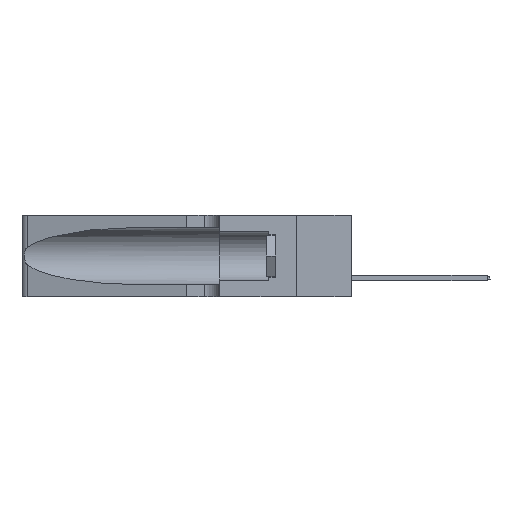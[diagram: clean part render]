
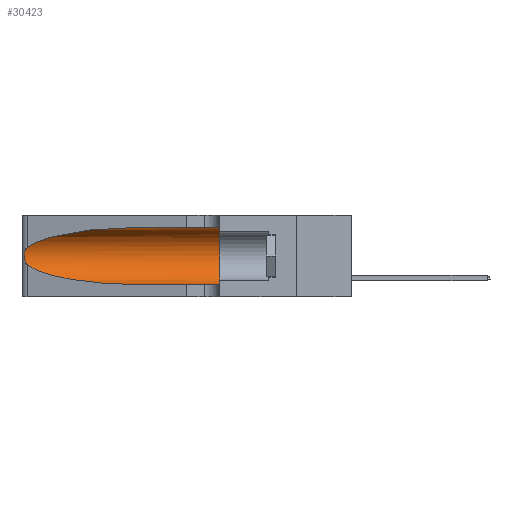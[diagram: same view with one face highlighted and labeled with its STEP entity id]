
A CAD part, left-side view. The second image highlights one B-rep face of the part: STEP entity #30423.
In plain terms, the highlighted cylindrical face has radius 3.308 mm (diameter 6.617 mm), a partial arc.
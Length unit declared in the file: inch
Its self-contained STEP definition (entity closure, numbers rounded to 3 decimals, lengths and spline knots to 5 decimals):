
#469 = VERTEX_POINT ( 'NONE', #9005 ) ;
#477 = CARTESIAN_POINT ( 'NONE',  ( 0.1305, 1.61858, 0.185 ) ) ;
#2237 = CARTESIAN_POINT ( 'NONE',  ( 0.1305, 0.72297, 0.31525 ) ) ;
#2876 = AXIS2_PLACEMENT_3D ( 'NONE', #477, #12611, #15053 ) ;
#3534 = CARTESIAN_POINT ( 'NONE',  ( 0.1305, 0.72297, 0.05475 ) ) ;
#3606 = CIRCLE ( 'NONE', #16011, 0.13025 ) ;
#4184 = CARTESIAN_POINT ( 'NONE',  ( 0.25555, 1.22993, 0.14849 ) ) ;
#4332 = CARTESIAN_POINT ( 'NONE',  ( 0.18966, 0.96281, 0.31525 ) ) ;
#4668 = CYLINDRICAL_SURFACE ( 'NONE', #2876, 0.13025 ) ;
#5025 = DIRECTION ( 'NONE',  ( 0., -1., 0. ) ) ;
#5222 = ORIENTED_EDGE ( 'NONE', *, *, #16551, .T. ) ;
#5290 = EDGE_CURVE ( 'NONE', #26591, #16849, #30680, .T. ) ;
#5317 = CARTESIAN_POINT ( 'NONE',  ( 0.25787, 1.23484, 0.2124 ) ) ;
#5686 = VECTOR ( 'NONE', #14224, 39.37008 ) ;
#5918 = B_SPLINE_CURVE_WITH_KNOTS ( 'NONE', 3,
 ( #22408, #17344, #20096, #5317, #20200, #22194, #24714, #27109, #20003, #15040, #16251, #17887, #4184, #11482 ),
 .UNSPECIFIED., .F., .F.,
 ( 4, 2, 2, 2, 2, 2, 4 ),
 ( 0., 0.00027, 0.00053, 0.00107, 0.0016, 0.00187, 0.00214 ),
 .UNSPECIFIED. ) ;
#6559 = EDGE_LOOP ( 'NONE', ( #10654, #5222, #26106, #30588, #6866, #19528 ) ) ;
#6730 = CARTESIAN_POINT ( 'NONE',  ( 0.1305, 1.61858, 0.05475 ) ) ;
#6866 = ORIENTED_EDGE ( 'NONE', *, *, #15186, .F. ) ;
#7002 = CARTESIAN_POINT ( 'NONE',  ( 0.1305, 0.35, 0.31525 ) ) ;
#8946 = DIRECTION ( 'NONE',  ( 0., 1., 0. ) ) ;
#9005 = CARTESIAN_POINT ( 'NONE',  ( 0.1305, 0.35, 0.05475 ) ) ;
#10654 = ORIENTED_EDGE ( 'NONE', *, *, #5290, .T. ) ;
#11482 = CARTESIAN_POINT ( 'NONE',  ( 0.25487, 1.22718, 0.14631 ) ) ;
#11954 = CARTESIAN_POINT ( 'NONE',  ( 0.25487, 1.22718, 0.14631 ) ) ;
#12048 = CARTESIAN_POINT ( 'NONE',  ( 0.2373, 1.15595, 0.08982 ) ) ;
#12611 = DIRECTION ( 'NONE',  ( 0., -1., 0. ) ) ;
#14224 = DIRECTION ( 'NONE',  ( 0., -1., 0. ) ) ;
#15040 = CARTESIAN_POINT ( 'NONE',  ( 0.25856, 1.23593, 0.16098 ) ) ;
#15053 = DIRECTION ( 'NONE',  ( 0., 0., -1. ) ) ;
#15186 = EDGE_CURVE ( 'NONE', #19406, #469, #3606, .T. ) ;
#16011 = AXIS2_PLACEMENT_3D ( 'NONE', #18134, #8946, #23082 ) ;
#16076 = LINE ( 'NONE', #19602, #28106 ) ;
#16251 = CARTESIAN_POINT ( 'NONE',  ( 0.25789, 1.23486, 0.15765 ) ) ;
#16551 = EDGE_CURVE ( 'NONE', #16849, #28461, #5918, .T. ) ;
#16686 = LINE ( 'NONE', #6730, #5686 ) ;
#16826 = CARTESIAN_POINT ( 'NONE',  ( 0.25487, 1.22718, 0.22369 ) ) ;
#16849 = VERTEX_POINT ( 'NONE', #16826 ) ;
#17171 = EDGE_CURVE ( 'NONE', #28461, #29223, #26404, .T. ) ;
#17344 = CARTESIAN_POINT ( 'NONE',  ( 0.25555, 1.22994, 0.2215 ) ) ;
#17887 = CARTESIAN_POINT ( 'NONE',  ( 0.25639, 1.23186, 0.15144 ) ) ;
#18134 = CARTESIAN_POINT ( 'NONE',  ( 0.1305, 0.35, 0.185 ) ) ;
#18818 = CARTESIAN_POINT ( 'NONE',  ( 0.1305, 0.72297, 0.31525 ) ) ;
#19406 = VERTEX_POINT ( 'NONE', #7002 ) ;
#19528 = ORIENTED_EDGE ( 'NONE', *, *, #26642, .F. ) ;
#19602 = CARTESIAN_POINT ( 'NONE',  ( 0.1305, 1.61858, 0.31525 ) ) ;
#20003 = CARTESIAN_POINT ( 'NONE',  ( 0.26017, 1.23833, 0.17102 ) ) ;
#20096 = CARTESIAN_POINT ( 'NONE',  ( 0.25639, 1.23184, 0.21858 ) ) ;
#20200 = CARTESIAN_POINT ( 'NONE',  ( 0.25854, 1.2359, 0.20912 ) ) ;
#21286 = FACE_OUTER_BOUND ( 'NONE', #6559, .T. ) ;
#21552 = CARTESIAN_POINT ( 'NONE',  ( 0.1305, 0.72297, 0.05475 ) ) ;
#21905 = EDGE_CURVE ( 'NONE', #29223, #469, #16686, .T. ) ;
#22194 = CARTESIAN_POINT ( 'NONE',  ( 0.26018, 1.23835, 0.19895 ) ) ;
#22408 = CARTESIAN_POINT ( 'NONE',  ( 0.25487, 1.22718, 0.22369 ) ) ;
#23052 = CARTESIAN_POINT ( 'NONE',  ( 0.25487, 1.22718, 0.14631 ) ) ;
#23082 = DIRECTION ( 'NONE',  ( 0., 0., 1. ) ) ;
#23249 = CARTESIAN_POINT ( 'NONE',  ( 0.25487, 1.22718, 0.22369 ) ) ;
#24714 = CARTESIAN_POINT ( 'NONE',  ( 0.26075, 1.23896, 0.19203 ) ) ;
#25768 = CARTESIAN_POINT ( 'NONE',  ( 0.2373, 1.15595, 0.28018 ) ) ;
#26106 = ORIENTED_EDGE ( 'NONE', *, *, #17171, .T. ) ;
#26404 =( BOUNDED_CURVE ( )  B_SPLINE_CURVE ( 3, ( #11954, #12048, #28894, #21552 ),
 .UNSPECIFIED., .F., .T. ) 
 B_SPLINE_CURVE_WITH_KNOTS ( ( 4, 4 ),
 ( 3.44316, 4.71239 ),
 .UNSPECIFIED. ) 
 CURVE ( )  GEOMETRIC_REPRESENTATION_ITEM ( )  RATIONAL_B_SPLINE_CURVE ( ( 1., 0.87, 0.87, 1. ) ) 
 REPRESENTATION_ITEM ( '' )  );
#26591 = VERTEX_POINT ( 'NONE', #2237 ) ;
#26642 = EDGE_CURVE ( 'NONE', #26591, #19406, #16076, .T. ) ;
#27109 = CARTESIAN_POINT ( 'NONE',  ( 0.26075, 1.23896, 0.178 ) ) ;
#28106 = VECTOR ( 'NONE', #5025, 39.37008 ) ;
#28461 = VERTEX_POINT ( 'NONE', #23052 ) ;
#28894 = CARTESIAN_POINT ( 'NONE',  ( 0.18966, 0.96281, 0.05475 ) ) ;
#29223 = VERTEX_POINT ( 'NONE', #3534 ) ;
#30423 = ADVANCED_FACE ( 'NONE', ( #21286 ), #4668, .F. ) ;
#30588 = ORIENTED_EDGE ( 'NONE', *, *, #21905, .T. ) ;
#30680 =( BOUNDED_CURVE ( )  B_SPLINE_CURVE ( 3, ( #18818, #4332, #25768, #23249 ),
 .UNSPECIFIED., .F., .F. ) 
 B_SPLINE_CURVE_WITH_KNOTS ( ( 4, 4 ),
 ( 1.5708, 2.84003 ),
 .UNSPECIFIED. ) 
 CURVE ( )  GEOMETRIC_REPRESENTATION_ITEM ( )  RATIONAL_B_SPLINE_CURVE ( ( 1., 0.87, 0.87, 1. ) ) 
 REPRESENTATION_ITEM ( '' )  );
